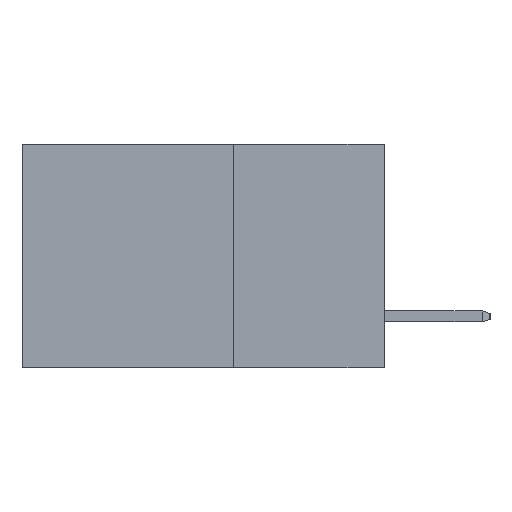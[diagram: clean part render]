
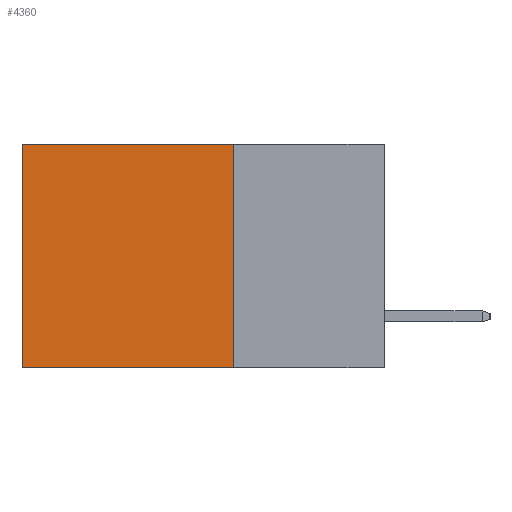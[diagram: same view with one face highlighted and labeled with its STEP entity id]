
A CAD part, left-side view. The second image highlights one B-rep face of the part: STEP entity #4360.
In plain terms, the highlighted planar face has unit normal (-1, 0, 0).
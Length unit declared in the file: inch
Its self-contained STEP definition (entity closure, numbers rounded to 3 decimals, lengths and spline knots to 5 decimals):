
#473 = LINE ( 'NONE', #684, #7652 ) ;
#492 = EDGE_CURVE ( 'NONE', #9073, #2210, #473, .T. ) ;
#649 = EDGE_CURVE ( 'NONE', #9073, #12140, #12847, .T. ) ;
#684 = CARTESIAN_POINT ( 'NONE',  ( 0.2615, 0.25, 0. ) ) ;
#1306 = AXIS2_PLACEMENT_3D ( 'NONE', #5809, #5785, #5721 ) ;
#2210 = VERTEX_POINT ( 'NONE', #7406 ) ;
#3371 = CARTESIAN_POINT ( 'NONE',  ( 0.2615, 0.25, -0.37 ) ) ;
#3385 = DIRECTION ( 'NONE',  ( 0., 1., 0. ) ) ;
#4360 = ADVANCED_FACE ( 'NONE', ( #16366 ), #5912, .F. ) ;
#4792 = VERTEX_POINT ( 'NONE', #13918 ) ;
#5423 = VECTOR ( 'NONE', #11545, 39.37008 ) ;
#5721 = DIRECTION ( 'NONE',  ( 0., 0., -1. ) ) ;
#5785 = DIRECTION ( 'NONE',  ( 1., 0., 0. ) ) ;
#5809 = CARTESIAN_POINT ( 'NONE',  ( 0.2615, 0.25, -0.37 ) ) ;
#5912 = PLANE ( 'NONE',  #1306 ) ;
#6425 = VECTOR ( 'NONE', #17996, 39.37008 ) ;
#7036 = LINE ( 'NONE', #15596, #10239 ) ;
#7406 = CARTESIAN_POINT ( 'NONE',  ( 0.2615, 0.6, 0. ) ) ;
#7652 = VECTOR ( 'NONE', #3385, 39.37008 ) ;
#7942 = ORIENTED_EDGE ( 'NONE', *, *, #649, .F. ) ;
#8546 = EDGE_CURVE ( 'NONE', #2210, #4792, #7036, .T. ) ;
#9073 = VERTEX_POINT ( 'NONE', #15233 ) ;
#9162 = EDGE_LOOP ( 'NONE', ( #9684, #9924, #7942, #14118 ) ) ;
#9684 = ORIENTED_EDGE ( 'NONE', *, *, #8546, .T. ) ;
#9924 = ORIENTED_EDGE ( 'NONE', *, *, #16294, .F. ) ;
#10239 = VECTOR ( 'NONE', #15798, 39.37008 ) ;
#11545 = DIRECTION ( 'NONE',  ( 0., 0., -1. ) ) ;
#11631 = CARTESIAN_POINT ( 'NONE',  ( 0.2615, 0.25, -0.37 ) ) ;
#12140 = VERTEX_POINT ( 'NONE', #3371 ) ;
#12847 = LINE ( 'NONE', #11631, #5423 ) ;
#13918 = CARTESIAN_POINT ( 'NONE',  ( 0.2615, 0.6, -0.37 ) ) ;
#14118 = ORIENTED_EDGE ( 'NONE', *, *, #492, .T. ) ;
#15233 = CARTESIAN_POINT ( 'NONE',  ( 0.2615, 0.25, 0. ) ) ;
#15596 = CARTESIAN_POINT ( 'NONE',  ( 0.2615, 0.6, -0.37 ) ) ;
#15798 = DIRECTION ( 'NONE',  ( 0., 0., -1. ) ) ;
#16144 = LINE ( 'NONE', #18053, #6425 ) ;
#16294 = EDGE_CURVE ( 'NONE', #12140, #4792, #16144, .T. ) ;
#16366 = FACE_OUTER_BOUND ( 'NONE', #9162, .T. ) ;
#17996 = DIRECTION ( 'NONE',  ( 0., 1., 0. ) ) ;
#18053 = CARTESIAN_POINT ( 'NONE',  ( 0.2615, 0.25, -0.37 ) ) ;
